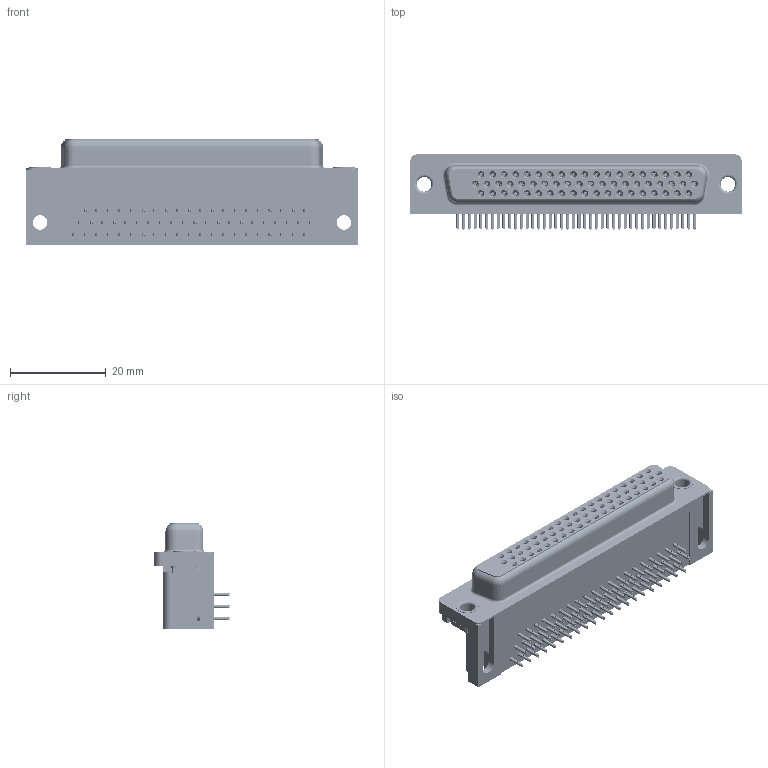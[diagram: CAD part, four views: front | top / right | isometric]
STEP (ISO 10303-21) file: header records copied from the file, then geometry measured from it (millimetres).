
FILE_DESCRIPTION (( 'STEP AP203' ), '1' );
FILE_NAME ('634-062-363-511.STEP', '2018-08-21T20:16:14', ( '' ), ( '' ), 'SwSTEP 2.0', 'SolidWorks 2016', '' );
FILE_SCHEMA (( 'CONFIG_CONTROL_DESIGN' ));
Length unit declared in the file: millimetre
Products named in the file (8): Thru Hole Board Mount; Thru Hole Rivet; 634-062-363-511; 634 Housing_62 Socket; 634 Shell_62 Socket; Contact Bottom; Contact Middle; Contact Top
Assembly tree (68 placements, depth 2):
  634-062-363-511
    634 Housing_62 Socket
    634 Shell_62 Socket
    Contact Bottom  x20
    Contact Middle  x21
    Contact Top  x21
    Thru Hole Board Mount  x2
    Thru Hole Rivet  x2
Bounding box: 69.4 x 15.73 x 22.1 mm (x, y, z)
Volume: 12930.1 mm3; surface area: 17720.7 mm2
Topology: 72 solids, 72 shells, 9055 faces, 23788 edges, 14922 vertices
Faces by surface type: plane 4089, bspline 2152, cylinder 2036, cone 744, torus 34
Entity records: 50504 total; most frequent: CARTESIAN_POINT 12979, ORIENTED_EDGE 7292, DIRECTION 6915, EDGE_CURVE 3646, LINE 2571, VECTOR 2571, VERTEX_POINT 2334, AXIS2_PLACEMENT_3D 2172
